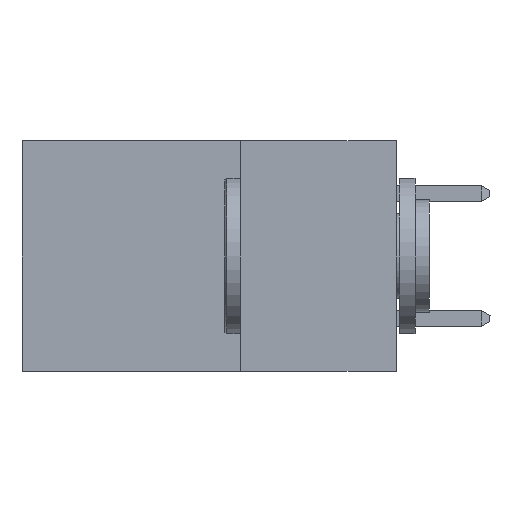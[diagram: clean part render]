
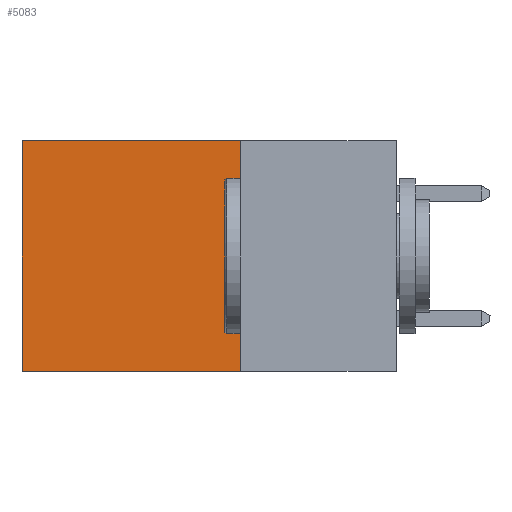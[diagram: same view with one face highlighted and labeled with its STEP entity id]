
A CAD part, left-side view. The second image highlights one B-rep face of the part: STEP entity #5083.
In plain terms, the highlighted planar face has unit normal (-1, 0, 0).
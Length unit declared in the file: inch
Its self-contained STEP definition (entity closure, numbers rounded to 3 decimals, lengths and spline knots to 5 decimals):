
#516 = EDGE_CURVE ( 'NONE', #8250, #1414, #1266, .T. ) ;
#1118 = EDGE_CURVE ( 'NONE', #1414, #10646, #3712, .T. ) ;
#1266 = LINE ( 'NONE', #7631, #13138 ) ;
#1414 = VERTEX_POINT ( 'NONE', #8067 ) ;
#1946 = VECTOR ( 'NONE', #12533, 39.37008 ) ;
#2270 = CARTESIAN_POINT ( 'NONE',  ( 0.2615, 0.25, 0. ) ) ;
#2604 = CARTESIAN_POINT ( 'NONE',  ( 0.2615, 0.25, 0. ) ) ;
#2746 = DIRECTION ( 'NONE',  ( 0., 0., -1. ) ) ;
#2772 = CARTESIAN_POINT ( 'NONE',  ( 0.2615, 0.6, -0.37 ) ) ;
#3023 = EDGE_LOOP ( 'NONE', ( #6753, #6859, #6874, #6941 ) ) ;
#3712 = LINE ( 'NONE', #4516, #9376 ) ;
#4516 = CARTESIAN_POINT ( 'NONE',  ( 0.2615, 0.25, -0.37 ) ) ;
#4831 = LINE ( 'NONE', #2772, #7532 ) ;
#5083 = ADVANCED_FACE ( 'NONE', ( #12692 ), #12094, .F. ) ;
#5182 = LINE ( 'NONE', #2270, #1946 ) ;
#5932 = DIRECTION ( 'NONE',  ( 0., 0., -1. ) ) ;
#5962 = DIRECTION ( 'NONE',  ( 0., 1., 0. ) ) ;
#6421 = AXIS2_PLACEMENT_3D ( 'NONE', #11838, #11872, #11810 ) ;
#6753 = ORIENTED_EDGE ( 'NONE', *, *, #12550, .T. ) ;
#6859 = ORIENTED_EDGE ( 'NONE', *, *, #1118, .F. ) ;
#6874 = ORIENTED_EDGE ( 'NONE', *, *, #516, .F. ) ;
#6941 = ORIENTED_EDGE ( 'NONE', *, *, #14342, .T. ) ;
#7532 = VECTOR ( 'NONE', #2746, 39.37008 ) ;
#7631 = CARTESIAN_POINT ( 'NONE',  ( 0.2615, 0.25, -0.37 ) ) ;
#8067 = CARTESIAN_POINT ( 'NONE',  ( 0.2615, 0.25, -0.37 ) ) ;
#8250 = VERTEX_POINT ( 'NONE', #2604 ) ;
#9174 = VERTEX_POINT ( 'NONE', #12841 ) ;
#9376 = VECTOR ( 'NONE', #5962, 39.37008 ) ;
#10646 = VERTEX_POINT ( 'NONE', #13540 ) ;
#11810 = DIRECTION ( 'NONE',  ( 0., 0., -1. ) ) ;
#11838 = CARTESIAN_POINT ( 'NONE',  ( 0.2615, 0.25, -0.37 ) ) ;
#11872 = DIRECTION ( 'NONE',  ( 1., 0., 0. ) ) ;
#12094 = PLANE ( 'NONE',  #6421 ) ;
#12533 = DIRECTION ( 'NONE',  ( 0., 1., 0. ) ) ;
#12550 = EDGE_CURVE ( 'NONE', #9174, #10646, #4831, .T. ) ;
#12692 = FACE_OUTER_BOUND ( 'NONE', #3023, .T. ) ;
#12841 = CARTESIAN_POINT ( 'NONE',  ( 0.2615, 0.6, 0. ) ) ;
#13138 = VECTOR ( 'NONE', #5932, 39.37008 ) ;
#13540 = CARTESIAN_POINT ( 'NONE',  ( 0.2615, 0.6, -0.37 ) ) ;
#14342 = EDGE_CURVE ( 'NONE', #8250, #9174, #5182, .T. ) ;
